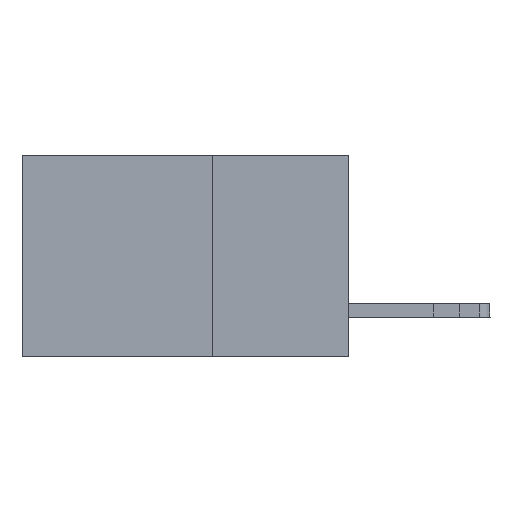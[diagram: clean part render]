
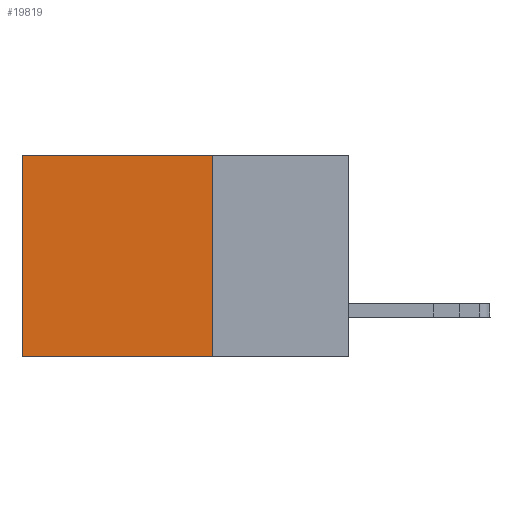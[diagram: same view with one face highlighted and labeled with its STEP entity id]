
A CAD part, left-side view. The second image highlights one B-rep face of the part: STEP entity #19819.
In plain terms, the highlighted planar face has unit normal (-1, 0, 0).
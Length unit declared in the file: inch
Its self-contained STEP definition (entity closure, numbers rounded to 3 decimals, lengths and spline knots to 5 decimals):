
#29 = CARTESIAN_POINT ( 'NONE',  ( 0.298, 0.25, -0.37 ) ) ;
#355 = DIRECTION ( 'NONE',  ( 0., 0., -1. ) ) ;
#470 = VECTOR ( 'NONE', #20284, 39.37008 ) ;
#2348 = FACE_OUTER_BOUND ( 'NONE', #6552, .T. ) ;
#2425 = ORIENTED_EDGE ( 'NONE', *, *, #11717, .T. ) ;
#2935 = VERTEX_POINT ( 'NONE', #25287 ) ;
#4852 = DIRECTION ( 'NONE',  ( 0., 0., -1. ) ) ;
#5117 = LINE ( 'NONE', #13217, #7001 ) ;
#5746 = CARTESIAN_POINT ( 'NONE',  ( 0.298, 0.25, -0.37 ) ) ;
#6552 = EDGE_LOOP ( 'NONE', ( #2425, #13386, #24121, #19994 ) ) ;
#7001 = VECTOR ( 'NONE', #4852, 39.37008 ) ;
#8130 = DIRECTION ( 'NONE',  ( 0., 1., 0. ) ) ;
#8195 = PLANE ( 'NONE',  #24801 ) ;
#11717 = EDGE_CURVE ( 'NONE', #21718, #2935, #20013, .T. ) ;
#11782 = VECTOR ( 'NONE', #8130, 39.37008 ) ;
#12613 = VERTEX_POINT ( 'NONE', #5746 ) ;
#13217 = CARTESIAN_POINT ( 'NONE',  ( 0.298, 0.25, 0. ) ) ;
#13386 = ORIENTED_EDGE ( 'NONE', *, *, #25914, .F. ) ;
#14610 = VECTOR ( 'NONE', #23838, 39.37008 ) ;
#16548 = CARTESIAN_POINT ( 'NONE',  ( 0.298, 0.25, 0. ) ) ;
#17724 = CARTESIAN_POINT ( 'NONE',  ( 0.298, 0.25, 0. ) ) ;
#18298 = CARTESIAN_POINT ( 'NONE',  ( 0.298, 0.6, 0. ) ) ;
#18648 = VERTEX_POINT ( 'NONE', #17724 ) ;
#19426 = CARTESIAN_POINT ( 'NONE',  ( 0.298, 0.6, 0. ) ) ;
#19819 = ADVANCED_FACE ( 'NONE', ( #2348 ), #8195, .F. ) ;
#19994 = ORIENTED_EDGE ( 'NONE', *, *, #22608, .T. ) ;
#19998 = EDGE_CURVE ( 'NONE', #18648, #12613, #5117, .T. ) ;
#20013 = LINE ( 'NONE', #18298, #470 ) ;
#20284 = DIRECTION ( 'NONE',  ( 0., 0., -1. ) ) ;
#21607 = CARTESIAN_POINT ( 'NONE',  ( 0.298, 0.25, 0. ) ) ;
#21718 = VERTEX_POINT ( 'NONE', #19426 ) ;
#22070 = LINE ( 'NONE', #29, #11782 ) ;
#22608 = EDGE_CURVE ( 'NONE', #18648, #21718, #23709, .T. ) ;
#23709 = LINE ( 'NONE', #21607, #14610 ) ;
#23838 = DIRECTION ( 'NONE',  ( 0., 1., 0. ) ) ;
#24121 = ORIENTED_EDGE ( 'NONE', *, *, #19998, .F. ) ;
#24658 = DIRECTION ( 'NONE',  ( 1., 0., 0. ) ) ;
#24801 = AXIS2_PLACEMENT_3D ( 'NONE', #16548, #24658, #355 ) ;
#25287 = CARTESIAN_POINT ( 'NONE',  ( 0.298, 0.6, -0.37 ) ) ;
#25914 = EDGE_CURVE ( 'NONE', #12613, #2935, #22070, .T. ) ;
